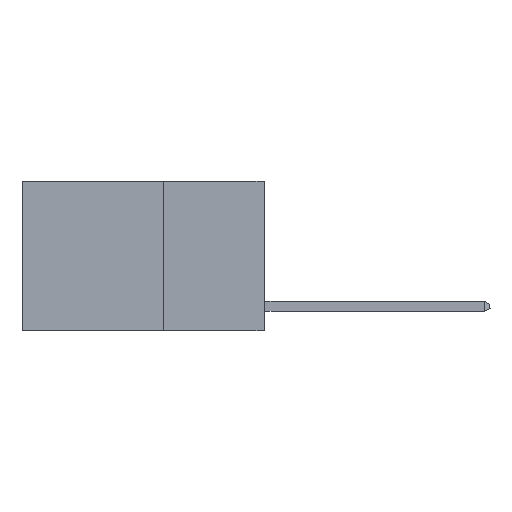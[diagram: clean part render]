
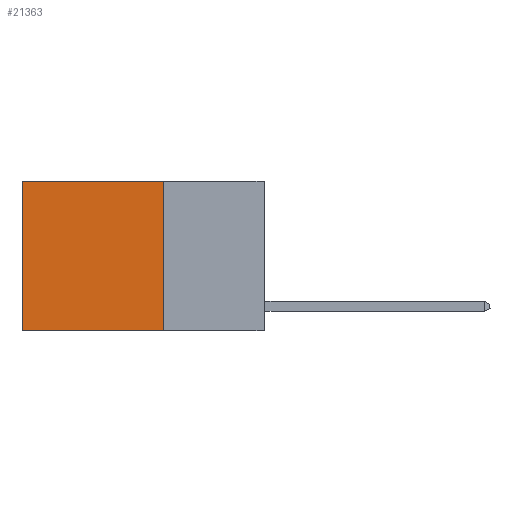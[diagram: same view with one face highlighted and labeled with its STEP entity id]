
A CAD part, left-side view. The second image highlights one B-rep face of the part: STEP entity #21363.
In plain terms, the highlighted planar face has unit normal (-1, 0, 0).
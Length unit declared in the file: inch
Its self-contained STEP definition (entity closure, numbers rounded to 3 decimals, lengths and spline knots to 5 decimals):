
#76 = CARTESIAN_POINT ( 'NONE',  ( 0.2625, 0.6, -0.37 ) ) ;
#435 = DIRECTION ( 'NONE',  ( 0., 0., -1. ) ) ;
#534 = LINE ( 'NONE', #14254, #18838 ) ;
#1026 = ORIENTED_EDGE ( 'NONE', *, *, #16611, .T. ) ;
#1205 = CARTESIAN_POINT ( 'NONE',  ( 0.2625, 0.25, 0. ) ) ;
#2167 = DIRECTION ( 'NONE',  ( 0., 1., 0. ) ) ;
#2218 = EDGE_LOOP ( 'NONE', ( #1026, #8424, #2698, #14985 ) ) ;
#2698 = ORIENTED_EDGE ( 'NONE', *, *, #13150, .F. ) ;
#2791 = VERTEX_POINT ( 'NONE', #6828 ) ;
#3243 = PLANE ( 'NONE',  #13967 ) ;
#3558 = EDGE_CURVE ( 'NONE', #14945, #2791, #534, .T. ) ;
#4548 = CARTESIAN_POINT ( 'NONE',  ( 0.2625, 0.25, -0.37 ) ) ;
#5013 = DIRECTION ( 'NONE',  ( 1., 0., 0. ) ) ;
#6193 = VECTOR ( 'NONE', #435, 39.37008 ) ;
#6417 = EDGE_CURVE ( 'NONE', #13528, #7313, #7315, .T. ) ;
#6828 = CARTESIAN_POINT ( 'NONE',  ( 0.2625, 0.6, 0. ) ) ;
#7313 = VERTEX_POINT ( 'NONE', #76 ) ;
#7315 = LINE ( 'NONE', #4548, #15300 ) ;
#8424 = ORIENTED_EDGE ( 'NONE', *, *, #6417, .F. ) ;
#9054 = FACE_OUTER_BOUND ( 'NONE', #2218, .T. ) ;
#10250 = LINE ( 'NONE', #10828, #6193 ) ;
#10418 = VECTOR ( 'NONE', #13321, 39.37008 ) ;
#10828 = CARTESIAN_POINT ( 'NONE',  ( 0.2625, 0.6, 0. ) ) ;
#10926 = LINE ( 'NONE', #1205, #10418 ) ;
#13150 = EDGE_CURVE ( 'NONE', #14945, #13528, #10926, .T. ) ;
#13321 = DIRECTION ( 'NONE',  ( 0., 0., -1. ) ) ;
#13528 = VERTEX_POINT ( 'NONE', #21065 ) ;
#13589 = CARTESIAN_POINT ( 'NONE',  ( 0.2625, 0.25, 0. ) ) ;
#13967 = AXIS2_PLACEMENT_3D ( 'NONE', #13589, #5013, #17002 ) ;
#14254 = CARTESIAN_POINT ( 'NONE',  ( 0.2625, 0.25, 0. ) ) ;
#14945 = VERTEX_POINT ( 'NONE', #21690 ) ;
#14985 = ORIENTED_EDGE ( 'NONE', *, *, #3558, .T. ) ;
#15300 = VECTOR ( 'NONE', #18241, 39.37008 ) ;
#16611 = EDGE_CURVE ( 'NONE', #2791, #7313, #10250, .T. ) ;
#17002 = DIRECTION ( 'NONE',  ( 0., 0., -1. ) ) ;
#18241 = DIRECTION ( 'NONE',  ( 0., 1., 0. ) ) ;
#18838 = VECTOR ( 'NONE', #2167, 39.37008 ) ;
#21065 = CARTESIAN_POINT ( 'NONE',  ( 0.2625, 0.25, -0.37 ) ) ;
#21363 = ADVANCED_FACE ( 'NONE', ( #9054 ), #3243, .F. ) ;
#21690 = CARTESIAN_POINT ( 'NONE',  ( 0.2625, 0.25, 0. ) ) ;
